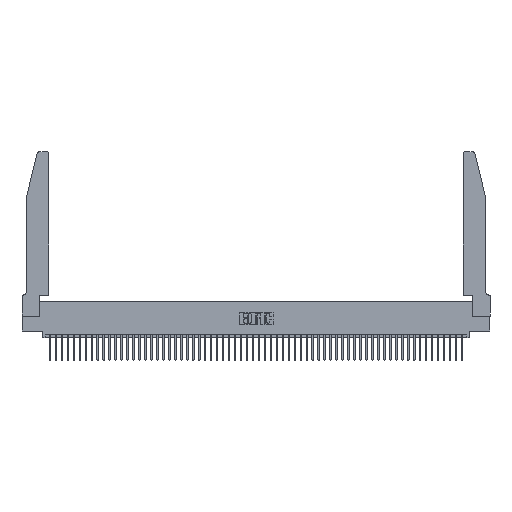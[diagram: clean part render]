
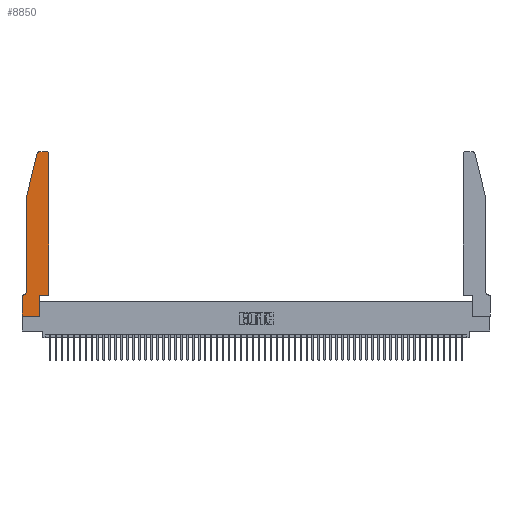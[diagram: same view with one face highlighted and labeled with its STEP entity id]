
A CAD part, top view. The second image highlights one B-rep face of the part: STEP entity #8850.
In plain terms, the highlighted planar face has unit normal (0, 0, 1).
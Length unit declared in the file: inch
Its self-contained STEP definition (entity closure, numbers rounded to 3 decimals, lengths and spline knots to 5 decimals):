
#39 = ORIENTED_EDGE ( 'NONE', *, *, #10982, .T. ) ;
#530 = CIRCLE ( 'NONE', #33964, 0.07 ) ;
#753 = VECTOR ( 'NONE', #40723, 39.37008 ) ;
#942 = CARTESIAN_POINT ( 'NONE',  ( 0.4505, 2.72, 0.37 ) ) ;
#1461 = DIRECTION ( 'NONE',  ( 1., 0., 0. ) ) ;
#1464 = ORIENTED_EDGE ( 'NONE', *, *, #32385, .T. ) ;
#2792 = CIRCLE ( 'NONE', #9315, 0.03 ) ;
#2894 = EDGE_CURVE ( 'NONE', #9025, #26416, #36969, .T. ) ;
#3392 = ORIENTED_EDGE ( 'NONE', *, *, #23752, .T. ) ;
#3643 = DIRECTION ( 'NONE',  ( 0., 0., 1. ) ) ;
#3688 = VERTEX_POINT ( 'NONE', #54650 ) ;
#4278 = DIRECTION ( 'NONE',  ( 1., 0., 0. ) ) ;
#5672 = CARTESIAN_POINT ( 'NONE',  ( 0.0055, 0.35, 0.37 ) ) ;
#5846 = ORIENTED_EDGE ( 'NONE', *, *, #42479, .T. ) ;
#5869 = CARTESIAN_POINT ( 'NONE',  ( 0., 0., 0.37 ) ) ;
#5982 = CARTESIAN_POINT ( 'NONE',  ( 0.2865, 0., 0.37 ) ) ;
#6130 = DIRECTION ( 'NONE',  ( 0., -1., 0. ) ) ;
#6251 = LINE ( 'NONE', #39823, #19345 ) ;
#6297 = AXIS2_PLACEMENT_3D ( 'NONE', #54849, #30406, #4278 ) ;
#7624 = CARTESIAN_POINT ( 'NONE',  ( 0.4205, 2.75, 0.37 ) ) ;
#8845 = VERTEX_POINT ( 'NONE', #48874 ) ;
#8850 = ADVANCED_FACE ( 'NONE', ( #47051 ), #49062, .T. ) ;
#9025 = VERTEX_POINT ( 'NONE', #11255 ) ;
#9309 = DIRECTION ( 'NONE',  ( 1., 0., 0. ) ) ;
#9315 = AXIS2_PLACEMENT_3D ( 'NONE', #29780, #3643, #34127 ) ;
#9967 = ORIENTED_EDGE ( 'NONE', *, *, #2894, .T. ) ;
#10982 = EDGE_CURVE ( 'NONE', #12785, #8845, #20524, .T. ) ;
#11255 = CARTESIAN_POINT ( 'NONE',  ( 0., 0.35, 0.37 ) ) ;
#12145 = ORIENTED_EDGE ( 'NONE', *, *, #24173, .T. ) ;
#12462 = LINE ( 'NONE', #45057, #753 ) ;
#12725 = CIRCLE ( 'NONE', #6297, 0.03 ) ;
#12785 = VERTEX_POINT ( 'NONE', #55670 ) ;
#12937 = VERTEX_POINT ( 'NONE', #52670 ) ;
#13451 = VERTEX_POINT ( 'NONE', #25734 ) ;
#14208 = VECTOR ( 'NONE', #16941, 39.37008 ) ;
#14767 = VECTOR ( 'NONE', #9309, 39.37008 ) ;
#14918 = ORIENTED_EDGE ( 'NONE', *, *, #42323, .T. ) ;
#15844 = CARTESIAN_POINT ( 'NONE',  ( 0.0055, 0.42, 0.37 ) ) ;
#15890 = ORIENTED_EDGE ( 'NONE', *, *, #55128, .T. ) ;
#16941 = DIRECTION ( 'NONE',  ( -1., 0., 0. ) ) ;
#17432 = DIRECTION ( 'NONE',  ( -0.239, -0.971, 0. ) ) ;
#17510 = ORIENTED_EDGE ( 'NONE', *, *, #50654, .T. ) ;
#18780 = VECTOR ( 'NONE', #34855, 39.37008 ) ;
#19237 = EDGE_CURVE ( 'NONE', #19526, #53682, #2792, .T. ) ;
#19345 = VECTOR ( 'NONE', #39644, 39.37008 ) ;
#19526 = VERTEX_POINT ( 'NONE', #942 ) ;
#20178 = LINE ( 'NONE', #49944, #28953 ) ;
#20251 = DIRECTION ( 'NONE',  ( -1., 0., 0. ) ) ;
#20524 = LINE ( 'NONE', #47567, #53469 ) ;
#20805 = VERTEX_POINT ( 'NONE', #5982 ) ;
#23345 = CARTESIAN_POINT ( 'NONE',  ( 0.284, 2.75, 0.37 ) ) ;
#23444 = EDGE_CURVE ( 'NONE', #12937, #3688, #32372, .T. ) ;
#23752 = EDGE_CURVE ( 'NONE', #35797, #9025, #20178, .T. ) ;
#24173 = EDGE_CURVE ( 'NONE', #26416, #20805, #41679, .T. ) ;
#25291 = CARTESIAN_POINT ( 'NONE',  ( 0.4505, 0.35, 0.37 ) ) ;
#25475 = VECTOR ( 'NONE', #6130, 39.37008 ) ;
#25717 = LINE ( 'NONE', #34146, #14208 ) ;
#25734 = CARTESIAN_POINT ( 'NONE',  ( 0.0755, 0.42, 0.37 ) ) ;
#26416 = VERTEX_POINT ( 'NONE', #5869 ) ;
#27614 = DIRECTION ( 'NONE',  ( 0., 0., 1. ) ) ;
#27854 = CARTESIAN_POINT ( 'NONE',  ( 0., 0., 0.37 ) ) ;
#27897 = LINE ( 'NONE', #25291, #50810 ) ;
#28571 = ORIENTED_EDGE ( 'NONE', *, *, #23444, .T. ) ;
#28953 = VECTOR ( 'NONE', #45259, 39.37008 ) ;
#29780 = CARTESIAN_POINT ( 'NONE',  ( 0.4205, 2.72, 0.37 ) ) ;
#30406 = DIRECTION ( 'NONE',  ( 0., 0., 1. ) ) ;
#32372 = LINE ( 'NONE', #35328, #14767 ) ;
#32385 = EDGE_CURVE ( 'NONE', #35200, #12785, #12725, .T. ) ;
#33964 = AXIS2_PLACEMENT_3D ( 'NONE', #15844, #46033, #20251 ) ;
#34127 = DIRECTION ( 'NONE',  ( 1., 0., 0. ) ) ;
#34146 = CARTESIAN_POINT ( 'NONE',  ( 0.2605, 2.75, 0.37 ) ) ;
#34761 = ORIENTED_EDGE ( 'NONE', *, *, #34859, .T. ) ;
#34855 = DIRECTION ( 'NONE',  ( 1., 0., 0. ) ) ;
#34859 = EDGE_CURVE ( 'NONE', #53682, #35200, #25717, .T. ) ;
#35200 = VERTEX_POINT ( 'NONE', #23345 ) ;
#35328 = CARTESIAN_POINT ( 'NONE',  ( 0.4505, 0.35, 0.37 ) ) ;
#35797 = VERTEX_POINT ( 'NONE', #5672 ) ;
#36969 = LINE ( 'NONE', #27854, #25475 ) ;
#39644 = DIRECTION ( 'NONE',  ( 0., -1., 0. ) ) ;
#39823 = CARTESIAN_POINT ( 'NONE',  ( 0.0755, 2., 0.37 ) ) ;
#40723 = DIRECTION ( 'NONE',  ( 0., 1., 0. ) ) ;
#41679 = LINE ( 'NONE', #51929, #18780 ) ;
#42323 = EDGE_CURVE ( 'NONE', #8845, #13451, #6251, .T. ) ;
#42479 = EDGE_CURVE ( 'NONE', #20805, #12937, #12462, .T. ) ;
#43686 = AXIS2_PLACEMENT_3D ( 'NONE', #53346, #27614, #1461 ) ;
#45057 = CARTESIAN_POINT ( 'NONE',  ( 0.2865, 0.35, 0.37 ) ) ;
#45259 = DIRECTION ( 'NONE',  ( -1., 0., 0. ) ) ;
#46033 = DIRECTION ( 'NONE',  ( 0., 0., -1. ) ) ;
#47051 = FACE_OUTER_BOUND ( 'NONE', #55980, .T. ) ;
#47567 = CARTESIAN_POINT ( 'NONE',  ( 0.0755, 2., 0.37 ) ) ;
#48874 = CARTESIAN_POINT ( 'NONE',  ( 0.0755, 2., 0.37 ) ) ;
#49062 = PLANE ( 'NONE',  #43686 ) ;
#49944 = CARTESIAN_POINT ( 'NONE',  ( 0.0755, 0.35, 0.37 ) ) ;
#50654 = EDGE_CURVE ( 'NONE', #3688, #19526, #27897, .T. ) ;
#50810 = VECTOR ( 'NONE', #51099, 39.37008 ) ;
#51099 = DIRECTION ( 'NONE',  ( 0., 1., 0. ) ) ;
#51929 = CARTESIAN_POINT ( 'NONE',  ( 0., 0., 0.37 ) ) ;
#52670 = CARTESIAN_POINT ( 'NONE',  ( 0.2865, 0.35, 0.37 ) ) ;
#53346 = CARTESIAN_POINT ( 'NONE',  ( 0., 0.35, 0.37 ) ) ;
#53469 = VECTOR ( 'NONE', #17432, 39.37008 ) ;
#53682 = VERTEX_POINT ( 'NONE', #7624 ) ;
#54650 = CARTESIAN_POINT ( 'NONE',  ( 0.4505, 0.35, 0.37 ) ) ;
#54849 = CARTESIAN_POINT ( 'NONE',  ( 0.284, 2.72, 0.37 ) ) ;
#55128 = EDGE_CURVE ( 'NONE', #13451, #35797, #530, .T. ) ;
#55670 = CARTESIAN_POINT ( 'NONE',  ( 0.25487, 2.72718, 0.37 ) ) ;
#55783 = ORIENTED_EDGE ( 'NONE', *, *, #19237, .T. ) ;
#55980 = EDGE_LOOP ( 'NONE', ( #34761, #1464, #39, #14918, #15890, #3392, #9967, #12145, #5846, #28571, #17510, #55783 ) ) ;
